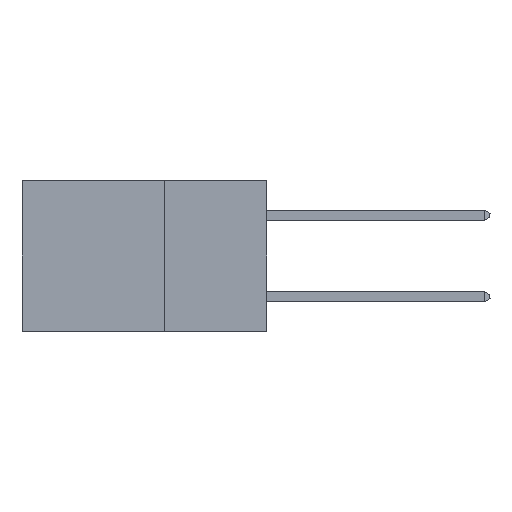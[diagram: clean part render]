
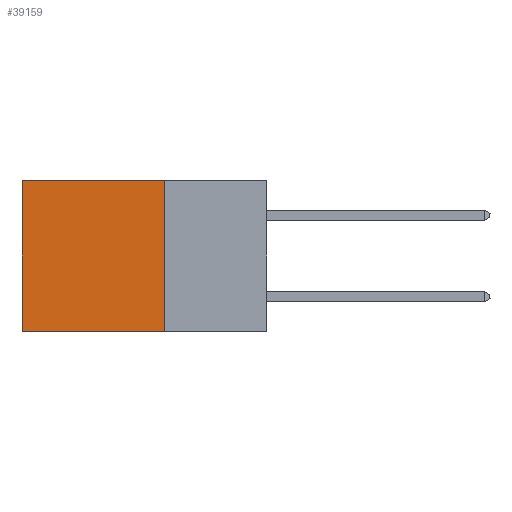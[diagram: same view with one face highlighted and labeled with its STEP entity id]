
A CAD part, left-side view. The second image highlights one B-rep face of the part: STEP entity #39159.
In plain terms, the highlighted planar face has unit normal (-1, 0, 0).
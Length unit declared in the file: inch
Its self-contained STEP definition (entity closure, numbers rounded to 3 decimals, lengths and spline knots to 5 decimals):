
#674 = ORIENTED_EDGE ( 'NONE', *, *, #38345, .T. ) ;
#4432 = EDGE_LOOP ( 'NONE', ( #24348, #11270, #10159, #674 ) ) ;
#5013 = CARTESIAN_POINT ( 'NONE',  ( 0.2875, 0.25, -0.37 ) ) ;
#8038 = DIRECTION ( 'NONE',  ( 0., 0., -1. ) ) ;
#8224 = DIRECTION ( 'NONE',  ( 0., 0., -1. ) ) ;
#8504 = VECTOR ( 'NONE', #29388, 39.37008 ) ;
#10159 = ORIENTED_EDGE ( 'NONE', *, *, #38501, .F. ) ;
#10862 = EDGE_CURVE ( 'NONE', #29184, #33401, #31320, .T. ) ;
#11270 = ORIENTED_EDGE ( 'NONE', *, *, #17638, .F. ) ;
#11706 = LINE ( 'NONE', #14872, #14211 ) ;
#14211 = VECTOR ( 'NONE', #8038, 39.37008 ) ;
#14872 = CARTESIAN_POINT ( 'NONE',  ( 0.2875, 0.25, 0. ) ) ;
#15992 = VERTEX_POINT ( 'NONE', #18560 ) ;
#16155 = CARTESIAN_POINT ( 'NONE',  ( 0.2875, 0.25, 0. ) ) ;
#17129 = VERTEX_POINT ( 'NONE', #34689 ) ;
#17638 = EDGE_CURVE ( 'NONE', #17129, #33401, #23846, .T. ) ;
#18011 = DIRECTION ( 'NONE',  ( 1., 0., 0. ) ) ;
#18305 = VECTOR ( 'NONE', #19410, 39.37008 ) ;
#18560 = CARTESIAN_POINT ( 'NONE',  ( 0.2875, 0.25, 0. ) ) ;
#19410 = DIRECTION ( 'NONE',  ( 0., 1., 0. ) ) ;
#23846 = LINE ( 'NONE', #5013, #30442 ) ;
#24348 = ORIENTED_EDGE ( 'NONE', *, *, #10862, .T. ) ;
#27644 = CARTESIAN_POINT ( 'NONE',  ( 0.2875, 0.25, 0. ) ) ;
#28400 = AXIS2_PLACEMENT_3D ( 'NONE', #27644, #18011, #8224 ) ;
#29184 = VERTEX_POINT ( 'NONE', #36937 ) ;
#29256 = CARTESIAN_POINT ( 'NONE',  ( 0.2875, 0.6, 0. ) ) ;
#29388 = DIRECTION ( 'NONE',  ( 0., 0., -1. ) ) ;
#30442 = VECTOR ( 'NONE', #40742, 39.37008 ) ;
#31320 = LINE ( 'NONE', #29256, #8504 ) ;
#33401 = VERTEX_POINT ( 'NONE', #37773 ) ;
#33971 = FACE_OUTER_BOUND ( 'NONE', #4432, .T. ) ;
#34689 = CARTESIAN_POINT ( 'NONE',  ( 0.2875, 0.25, -0.37 ) ) ;
#35024 = LINE ( 'NONE', #16155, #18305 ) ;
#36937 = CARTESIAN_POINT ( 'NONE',  ( 0.2875, 0.6, 0. ) ) ;
#37773 = CARTESIAN_POINT ( 'NONE',  ( 0.2875, 0.6, -0.37 ) ) ;
#38345 = EDGE_CURVE ( 'NONE', #15992, #29184, #35024, .T. ) ;
#38501 = EDGE_CURVE ( 'NONE', #15992, #17129, #11706, .T. ) ;
#39159 = ADVANCED_FACE ( 'NONE', ( #33971 ), #40544, .F. ) ;
#40544 = PLANE ( 'NONE',  #28400 ) ;
#40742 = DIRECTION ( 'NONE',  ( 0., 1., 0. ) ) ;
